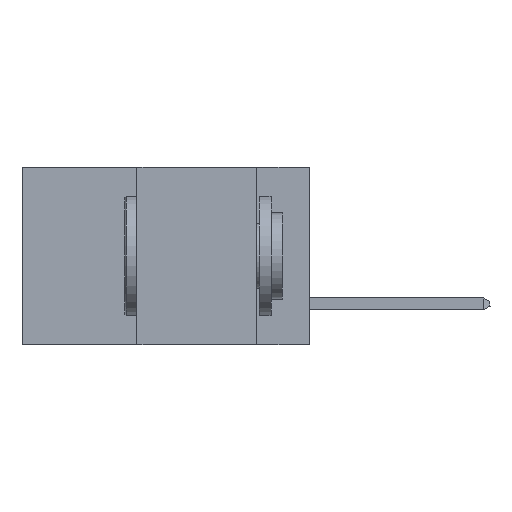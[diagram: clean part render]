
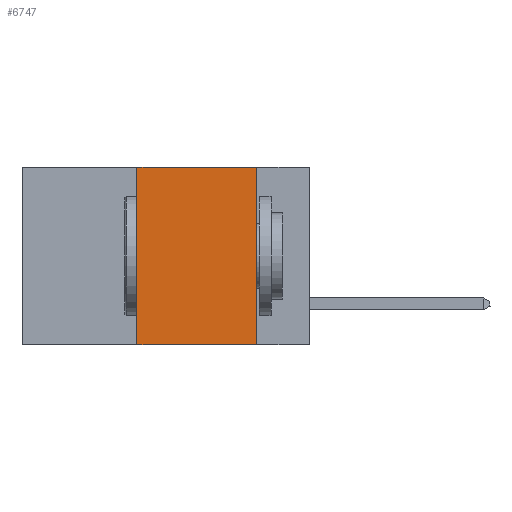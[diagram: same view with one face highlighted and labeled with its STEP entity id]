
A CAD part, left-side view. The second image highlights one B-rep face of the part: STEP entity #6747.
In plain terms, the highlighted planar face has unit normal (-1, 0, 0).
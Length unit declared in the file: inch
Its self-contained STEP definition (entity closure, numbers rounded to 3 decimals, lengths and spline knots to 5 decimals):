
#620 = LINE ( 'NONE', #25847, #23466 ) ;
#835 = FACE_OUTER_BOUND ( 'NONE', #15496, .T. ) ;
#1445 = CARTESIAN_POINT ( 'NONE',  ( 0., 0.11, 0. ) ) ;
#4478 = ORIENTED_EDGE ( 'NONE', *, *, #30340, .T. ) ;
#4874 = VERTEX_POINT ( 'NONE', #33036 ) ;
#6747 = ADVANCED_FACE ( 'NONE', ( #835 ), #23846, .F. ) ;
#7945 = VERTEX_POINT ( 'NONE', #18603 ) ;
#9036 = VECTOR ( 'NONE', #19496, 39.37008 ) ;
#9471 = VECTOR ( 'NONE', #16733, 39.37008 ) ;
#11716 = DIRECTION ( 'NONE',  ( 1., 0., 0. ) ) ;
#14516 = DIRECTION ( 'NONE',  ( 0., 0., -1. ) ) ;
#14536 = EDGE_CURVE ( 'NONE', #23192, #4874, #28457, .T. ) ;
#14763 = EDGE_CURVE ( 'NONE', #27333, #7945, #35986, .T. ) ;
#15496 = EDGE_LOOP ( 'NONE', ( #19444, #20596, #24787, #4478 ) ) ;
#16295 = AXIS2_PLACEMENT_3D ( 'NONE', #30003, #11716, #14516 ) ;
#16733 = DIRECTION ( 'NONE',  ( 0., 0., -1. ) ) ;
#17121 = VECTOR ( 'NONE', #20145, 39.37008 ) ;
#18603 = CARTESIAN_POINT ( 'NONE',  ( 0., 0.11, -0.37 ) ) ;
#19444 = ORIENTED_EDGE ( 'NONE', *, *, #14763, .F. ) ;
#19496 = DIRECTION ( 'NONE',  ( 0., 0., 1. ) ) ;
#19790 = EDGE_CURVE ( 'NONE', #4874, #27333, #32682, .T. ) ;
#20145 = DIRECTION ( 'NONE',  ( 0., -1., 0. ) ) ;
#20596 = ORIENTED_EDGE ( 'NONE', *, *, #19790, .F. ) ;
#22573 = CARTESIAN_POINT ( 'NONE',  ( 0., 0.6, 0. ) ) ;
#22588 = CARTESIAN_POINT ( 'NONE',  ( 0., 0.36, 0. ) ) ;
#23192 = VERTEX_POINT ( 'NONE', #38643 ) ;
#23466 = VECTOR ( 'NONE', #34495, 39.37008 ) ;
#23846 = PLANE ( 'NONE',  #16295 ) ;
#24787 = ORIENTED_EDGE ( 'NONE', *, *, #14536, .F. ) ;
#25038 = CARTESIAN_POINT ( 'NONE',  ( 0., 0.11, 0. ) ) ;
#25847 = CARTESIAN_POINT ( 'NONE',  ( 0., 0.6, -0.37 ) ) ;
#27333 = VERTEX_POINT ( 'NONE', #25038 ) ;
#28457 = LINE ( 'NONE', #22588, #9036 ) ;
#30003 = CARTESIAN_POINT ( 'NONE',  ( 0., 0.6, 0. ) ) ;
#30340 = EDGE_CURVE ( 'NONE', #23192, #7945, #620, .T. ) ;
#32682 = LINE ( 'NONE', #22573, #17121 ) ;
#33036 = CARTESIAN_POINT ( 'NONE',  ( 0., 0.36, 0. ) ) ;
#34495 = DIRECTION ( 'NONE',  ( 0., -1., 0. ) ) ;
#35986 = LINE ( 'NONE', #1445, #9471 ) ;
#38643 = CARTESIAN_POINT ( 'NONE',  ( 0., 0.36, -0.37 ) ) ;
